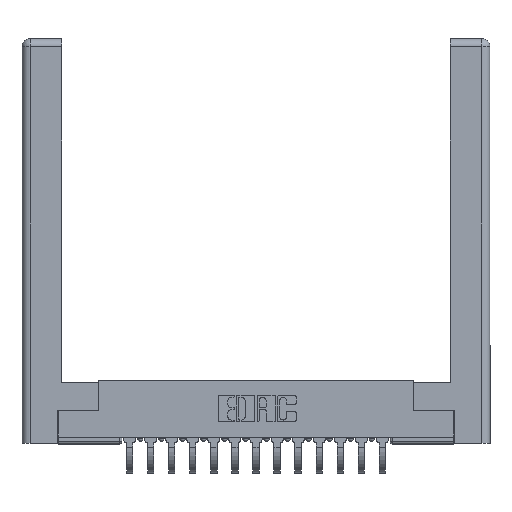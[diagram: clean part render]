
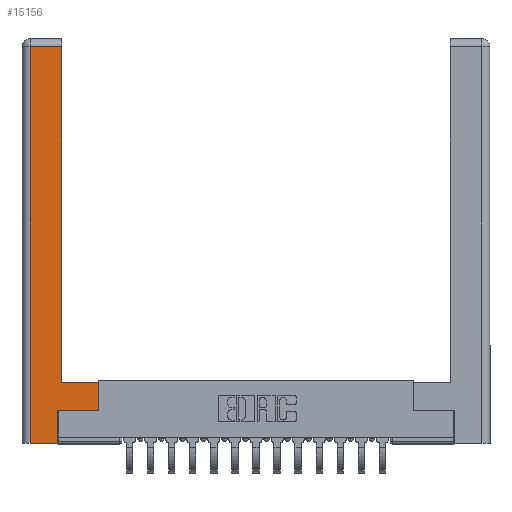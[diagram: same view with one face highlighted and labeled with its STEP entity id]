
A CAD part, top view. The second image highlights one B-rep face of the part: STEP entity #15156.
In plain terms, the highlighted planar face has unit normal (0, 0, 1).
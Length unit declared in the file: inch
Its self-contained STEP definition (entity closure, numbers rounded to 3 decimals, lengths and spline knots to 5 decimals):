
#537 = DIRECTION ( 'NONE',  ( 1., 0., 0. ) ) ;
#668 = CARTESIAN_POINT ( 'NONE',  ( 0.565, 0.45, 0. ) ) ;
#1721 = DIRECTION ( 'NONE',  ( -1., 0., 0. ) ) ;
#2291 = LINE ( 'NONE', #9896, #17025 ) ;
#2765 = EDGE_CURVE ( 'NONE', #12883, #6962, #3409, .T. ) ;
#2800 = CARTESIAN_POINT ( 'NONE',  ( 0.0615, 2.94, 0. ) ) ;
#3301 = LINE ( 'NONE', #7793, #4080 ) ;
#3409 = LINE ( 'NONE', #7804, #6983 ) ;
#3971 = DIRECTION ( 'NONE',  ( -1., 0., 0. ) ) ;
#4080 = VECTOR ( 'NONE', #15388, 39.37008 ) ;
#4645 = DIRECTION ( 'NONE',  ( 0., 0., -1. ) ) ;
#4857 = VECTOR ( 'NONE', #5425, 39.37008 ) ;
#4905 = EDGE_CURVE ( 'NONE', #13129, #5543, #6069, .T. ) ;
#5051 = VERTEX_POINT ( 'NONE', #18762 ) ;
#5341 = LINE ( 'NONE', #668, #12773 ) ;
#5425 = DIRECTION ( 'NONE',  ( 0., -1., 0. ) ) ;
#5456 = CARTESIAN_POINT ( 'NONE',  ( 0.565, 0.45, 0. ) ) ;
#5543 = VERTEX_POINT ( 'NONE', #9616 ) ;
#5827 = EDGE_CURVE ( 'NONE', #5543, #8354, #15048, .T. ) ;
#5884 = CARTESIAN_POINT ( 'NONE',  ( 0.265, 0., 0. ) ) ;
#6000 = VERTEX_POINT ( 'NONE', #9291 ) ;
#6069 = LINE ( 'NONE', #11752, #12403 ) ;
#6125 = FACE_OUTER_BOUND ( 'NONE', #10761, .T. ) ;
#6193 = CARTESIAN_POINT ( 'NONE',  ( 0.295, 3., 0. ) ) ;
#6308 = PLANE ( 'NONE',  #7486 ) ;
#6653 = VECTOR ( 'NONE', #3971, 39.37008 ) ;
#6962 = VERTEX_POINT ( 'NONE', #14131 ) ;
#6983 = VECTOR ( 'NONE', #13946, 39.37008 ) ;
#7002 = CARTESIAN_POINT ( 'NONE',  ( 0.0615, 0., 0. ) ) ;
#7486 = AXIS2_PLACEMENT_3D ( 'NONE', #18171, #4645, #1721 ) ;
#7793 = CARTESIAN_POINT ( 'NONE',  ( 0.265, 0., 0. ) ) ;
#7804 = CARTESIAN_POINT ( 'NONE',  ( 0.265, 0.245, 0. ) ) ;
#8179 = DIRECTION ( 'NONE',  ( 0., 1., 0. ) ) ;
#8260 = VERTEX_POINT ( 'NONE', #18772 ) ;
#8354 = VERTEX_POINT ( 'NONE', #12744 ) ;
#8715 = EDGE_CURVE ( 'NONE', #6000, #8260, #9818, .T. ) ;
#9093 = EDGE_CURVE ( 'NONE', #6962, #5051, #2291, .T. ) ;
#9291 = CARTESIAN_POINT ( 'NONE',  ( 0.0615, 2.94, 0. ) ) ;
#9616 = CARTESIAN_POINT ( 'NONE',  ( 0.295, 0.45, 0. ) ) ;
#9818 = LINE ( 'NONE', #7002, #4857 ) ;
#9896 = CARTESIAN_POINT ( 'NONE',  ( 0.565, 0.245, 0. ) ) ;
#10247 = ORIENTED_EDGE ( 'NONE', *, *, #2765, .T. ) ;
#10557 = DIRECTION ( 'NONE',  ( -1., 0., 0. ) ) ;
#10761 = EDGE_LOOP ( 'NONE', ( #14201, #13214, #13313, #13731, #10247, #16858, #14805, #11186 ) ) ;
#10841 = VECTOR ( 'NONE', #14956, 39.37008 ) ;
#11186 = ORIENTED_EDGE ( 'NONE', *, *, #4905, .T. ) ;
#11752 = CARTESIAN_POINT ( 'NONE',  ( 0.295, 0.45, 0. ) ) ;
#12403 = VECTOR ( 'NONE', #10557, 39.37008 ) ;
#12744 = CARTESIAN_POINT ( 'NONE',  ( 0.295, 2.94, 0. ) ) ;
#12773 = VECTOR ( 'NONE', #8179, 39.37008 ) ;
#12883 = VERTEX_POINT ( 'NONE', #5884 ) ;
#13129 = VERTEX_POINT ( 'NONE', #5456 ) ;
#13214 = ORIENTED_EDGE ( 'NONE', *, *, #18687, .T. ) ;
#13313 = ORIENTED_EDGE ( 'NONE', *, *, #8715, .T. ) ;
#13731 = ORIENTED_EDGE ( 'NONE', *, *, #16084, .T. ) ;
#13946 = DIRECTION ( 'NONE',  ( 0., 1., 0. ) ) ;
#14131 = CARTESIAN_POINT ( 'NONE',  ( 0.265, 0.245, 0. ) ) ;
#14201 = ORIENTED_EDGE ( 'NONE', *, *, #5827, .T. ) ;
#14805 = ORIENTED_EDGE ( 'NONE', *, *, #14906, .T. ) ;
#14906 = EDGE_CURVE ( 'NONE', #5051, #13129, #5341, .T. ) ;
#14956 = DIRECTION ( 'NONE',  ( 0., 1., 0. ) ) ;
#15048 = LINE ( 'NONE', #6193, #10841 ) ;
#15156 = ADVANCED_FACE ( 'NONE', ( #6125 ), #6308, .F. ) ;
#15388 = DIRECTION ( 'NONE',  ( 1., 0., 0. ) ) ;
#16084 = EDGE_CURVE ( 'NONE', #8260, #12883, #3301, .T. ) ;
#16858 = ORIENTED_EDGE ( 'NONE', *, *, #9093, .T. ) ;
#17025 = VECTOR ( 'NONE', #537, 39.37008 ) ;
#18171 = CARTESIAN_POINT ( 'NONE',  ( 0., 0., 0. ) ) ;
#18687 = EDGE_CURVE ( 'NONE', #8354, #6000, #19235, .T. ) ;
#18762 = CARTESIAN_POINT ( 'NONE',  ( 0.565, 0.245, 0. ) ) ;
#18772 = CARTESIAN_POINT ( 'NONE',  ( 0.0615, 0., 0. ) ) ;
#19235 = LINE ( 'NONE', #2800, #6653 ) ;
